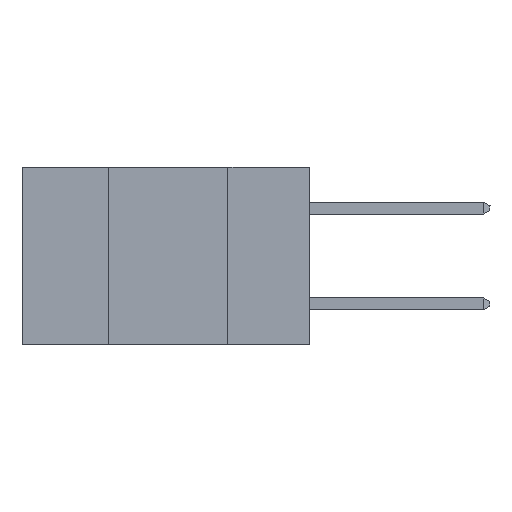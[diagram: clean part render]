
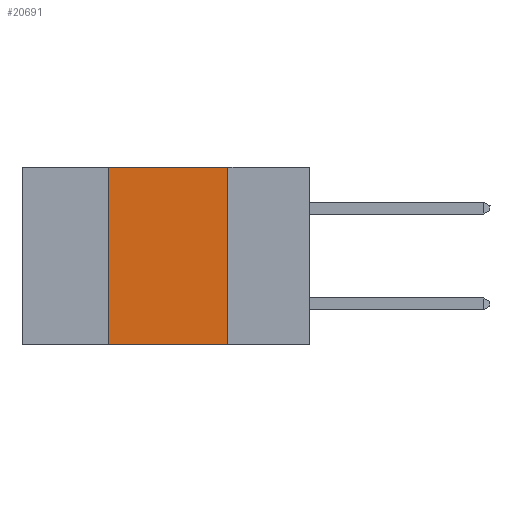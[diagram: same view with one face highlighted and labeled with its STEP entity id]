
A CAD part, left-side view. The second image highlights one B-rep face of the part: STEP entity #20691.
In plain terms, the highlighted planar face has unit normal (-1, 0, 0).
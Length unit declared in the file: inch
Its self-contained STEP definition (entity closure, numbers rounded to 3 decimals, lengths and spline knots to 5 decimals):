
#958 = ORIENTED_EDGE ( 'NONE', *, *, #16219, .F. ) ;
#1251 = CARTESIAN_POINT ( 'NONE',  ( 0., 0.17, 0. ) ) ;
#2021 = CARTESIAN_POINT ( 'NONE',  ( 0., 0.6, 0. ) ) ;
#2264 = PLANE ( 'NONE',  #3955 ) ;
#2396 = EDGE_CURVE ( 'NONE', #13231, #7638, #20141, .T. ) ;
#2829 = DIRECTION ( 'NONE',  ( 0., 0., 1. ) ) ;
#3230 = CARTESIAN_POINT ( 'NONE',  ( 0., 0.42, 0. ) ) ;
#3955 = AXIS2_PLACEMENT_3D ( 'NONE', #18513, #7841, #20267 ) ;
#4352 = CARTESIAN_POINT ( 'NONE',  ( 0., 0.17, 0. ) ) ;
#4715 = CARTESIAN_POINT ( 'NONE',  ( 0., 0.42, 0. ) ) ;
#4922 = LINE ( 'NONE', #4715, #18661 ) ;
#5031 = VERTEX_POINT ( 'NONE', #3230 ) ;
#5930 = VECTOR ( 'NONE', #6786, 39.37008 ) ;
#6710 = CARTESIAN_POINT ( 'NONE',  ( 0., 0.6, -0.37 ) ) ;
#6786 = DIRECTION ( 'NONE',  ( 0., -1., 0. ) ) ;
#7638 = VERTEX_POINT ( 'NONE', #8496 ) ;
#7841 = DIRECTION ( 'NONE',  ( 1., 0., 0. ) ) ;
#8496 = CARTESIAN_POINT ( 'NONE',  ( 0., 0.17, -0.37 ) ) ;
#9578 = ORIENTED_EDGE ( 'NONE', *, *, #20576, .F. ) ;
#10438 = VECTOR ( 'NONE', #14732, 39.37008 ) ;
#11837 = CARTESIAN_POINT ( 'NONE',  ( 0., 0.42, -0.37 ) ) ;
#12405 = FACE_OUTER_BOUND ( 'NONE', #18938, .T. ) ;
#13231 = VERTEX_POINT ( 'NONE', #11837 ) ;
#14621 = LINE ( 'NONE', #2021, #10438 ) ;
#14732 = DIRECTION ( 'NONE',  ( 0., -1., 0. ) ) ;
#15766 = VERTEX_POINT ( 'NONE', #1251 ) ;
#16005 = ORIENTED_EDGE ( 'NONE', *, *, #2396, .T. ) ;
#16219 = EDGE_CURVE ( 'NONE', #13231, #5031, #4922, .T. ) ;
#18480 = ORIENTED_EDGE ( 'NONE', *, *, #18862, .F. ) ;
#18513 = CARTESIAN_POINT ( 'NONE',  ( 0., 0.6, 0. ) ) ;
#18661 = VECTOR ( 'NONE', #2829, 39.37008 ) ;
#18728 = DIRECTION ( 'NONE',  ( 0., 0., -1. ) ) ;
#18830 = LINE ( 'NONE', #4352, #22922 ) ;
#18862 = EDGE_CURVE ( 'NONE', #15766, #7638, #18830, .T. ) ;
#18938 = EDGE_LOOP ( 'NONE', ( #18480, #9578, #958, #16005 ) ) ;
#20141 = LINE ( 'NONE', #6710, #5930 ) ;
#20267 = DIRECTION ( 'NONE',  ( 0., 0., -1. ) ) ;
#20576 = EDGE_CURVE ( 'NONE', #5031, #15766, #14621, .T. ) ;
#20691 = ADVANCED_FACE ( 'NONE', ( #12405 ), #2264, .F. ) ;
#22922 = VECTOR ( 'NONE', #18728, 39.37008 ) ;
